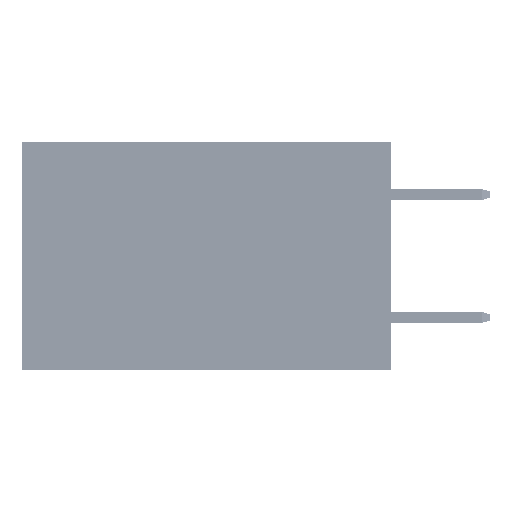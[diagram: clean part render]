
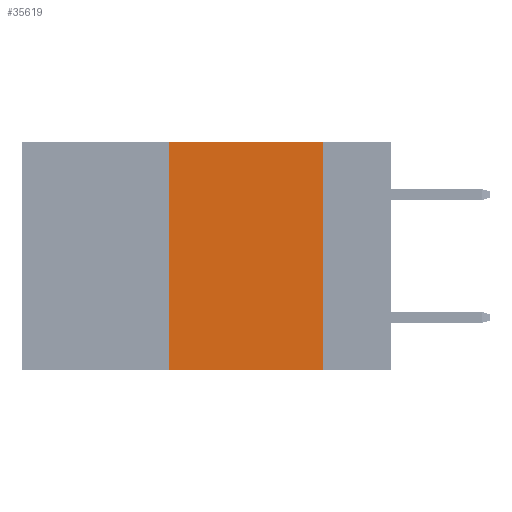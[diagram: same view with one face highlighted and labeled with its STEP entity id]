
A CAD part, left-side view. The second image highlights one B-rep face of the part: STEP entity #35619.
In plain terms, the highlighted planar face has unit normal (-1, 0, 0).
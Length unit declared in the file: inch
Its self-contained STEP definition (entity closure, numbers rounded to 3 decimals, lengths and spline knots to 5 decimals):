
#715 = VERTEX_POINT ( 'NONE', #20728 ) ;
#2503 = EDGE_CURVE ( 'NONE', #43663, #22173, #36973, .T. ) ;
#2617 = VECTOR ( 'NONE', #31626, 39.37008 ) ;
#5180 = PLANE ( 'NONE',  #47666 ) ;
#5337 = EDGE_CURVE ( 'NONE', #715, #43663, #16477, .T. ) ;
#8891 = CARTESIAN_POINT ( 'NONE',  ( 0., 0.36, 0. ) ) ;
#8962 = ORIENTED_EDGE ( 'NONE', *, *, #5337, .F. ) ;
#10457 = VECTOR ( 'NONE', #30892, 39.37008 ) ;
#11807 = CARTESIAN_POINT ( 'NONE',  ( 0., 0.6, 0. ) ) ;
#12381 = CARTESIAN_POINT ( 'NONE',  ( 0., 0.6, 0. ) ) ;
#12707 = DIRECTION ( 'NONE',  ( 0., 0., -1. ) ) ;
#13083 = EDGE_LOOP ( 'NONE', ( #16612, #8962, #28679, #21827 ) ) ;
#14105 = VECTOR ( 'NONE', #24145, 39.37008 ) ;
#16246 = CARTESIAN_POINT ( 'NONE',  ( 0., 0.6, -0.37 ) ) ;
#16358 = CARTESIAN_POINT ( 'NONE',  ( 0., 0.11, -0.37 ) ) ;
#16477 = LINE ( 'NONE', #11807, #14105 ) ;
#16612 = ORIENTED_EDGE ( 'NONE', *, *, #2503, .F. ) ;
#19242 = CARTESIAN_POINT ( 'NONE',  ( 0., 0.11, 0. ) ) ;
#20728 = CARTESIAN_POINT ( 'NONE',  ( 0., 0.36, 0. ) ) ;
#21827 = ORIENTED_EDGE ( 'NONE', *, *, #23498, .T. ) ;
#22173 = VERTEX_POINT ( 'NONE', #16358 ) ;
#23284 = VERTEX_POINT ( 'NONE', #26652 ) ;
#23498 = EDGE_CURVE ( 'NONE', #23284, #22173, #36653, .T. ) ;
#24145 = DIRECTION ( 'NONE',  ( 0., -1., 0. ) ) ;
#25253 = VECTOR ( 'NONE', #27242, 39.37008 ) ;
#26652 = CARTESIAN_POINT ( 'NONE',  ( 0., 0.36, -0.37 ) ) ;
#27242 = DIRECTION ( 'NONE',  ( 0., 0., 1. ) ) ;
#28679 = ORIENTED_EDGE ( 'NONE', *, *, #33111, .F. ) ;
#30892 = DIRECTION ( 'NONE',  ( 0., -1., 0. ) ) ;
#31626 = DIRECTION ( 'NONE',  ( 0., 0., -1. ) ) ;
#33111 = EDGE_CURVE ( 'NONE', #23284, #715, #41565, .T. ) ;
#35619 = ADVANCED_FACE ( 'NONE', ( #44828 ), #5180, .F. ) ;
#36653 = LINE ( 'NONE', #16246, #10457 ) ;
#36973 = LINE ( 'NONE', #46228, #2617 ) ;
#38722 = DIRECTION ( 'NONE',  ( 1., 0., 0. ) ) ;
#41565 = LINE ( 'NONE', #8891, #25253 ) ;
#43663 = VERTEX_POINT ( 'NONE', #19242 ) ;
#44828 = FACE_OUTER_BOUND ( 'NONE', #13083, .T. ) ;
#46228 = CARTESIAN_POINT ( 'NONE',  ( 0., 0.11, 0. ) ) ;
#47666 = AXIS2_PLACEMENT_3D ( 'NONE', #12381, #38722, #12707 ) ;
